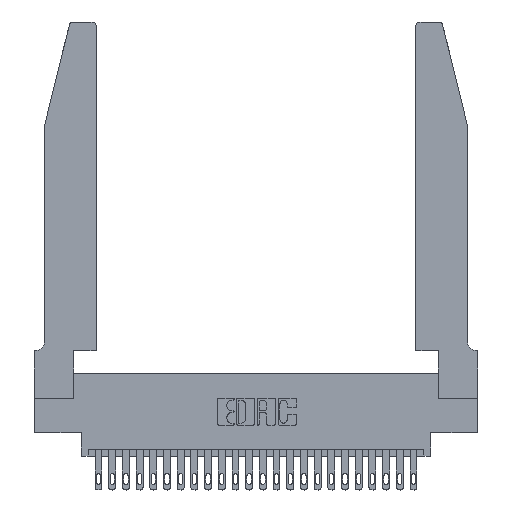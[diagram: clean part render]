
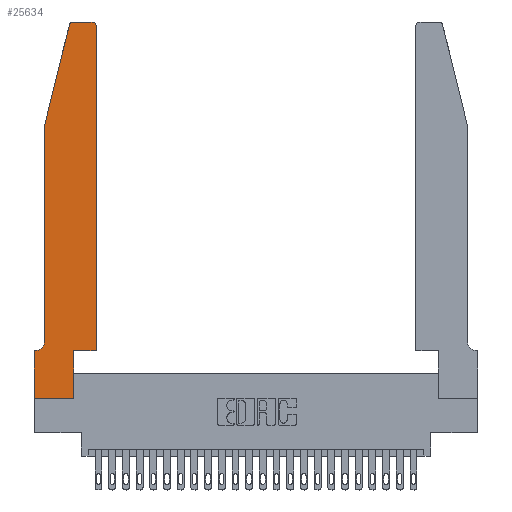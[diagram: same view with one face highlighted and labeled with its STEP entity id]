
A CAD part, top view. The second image highlights one B-rep face of the part: STEP entity #25634.
In plain terms, the highlighted planar face has unit normal (0, 0, 1).
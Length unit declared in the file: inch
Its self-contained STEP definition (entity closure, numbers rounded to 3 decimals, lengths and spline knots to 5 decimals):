
#237 = PLANE ( 'NONE',  #3318 ) ;
#264 = LINE ( 'NONE', #15603, #20413 ) ;
#269 = VERTEX_POINT ( 'NONE', #1125 ) ;
#281 = EDGE_CURVE ( 'NONE', #613, #19661, #6562, .T. ) ;
#613 = VERTEX_POINT ( 'NONE', #22108 ) ;
#935 = FACE_OUTER_BOUND ( 'NONE', #7405, .T. ) ;
#1125 = CARTESIAN_POINT ( 'NONE',  ( 0.2865, 0.35, 0.37 ) ) ;
#1539 = ORIENTED_EDGE ( 'NONE', *, *, #22946, .T. ) ;
#1851 = DIRECTION ( 'NONE',  ( -1., 0., 0. ) ) ;
#2053 = DIRECTION ( 'NONE',  ( 0., 0., 1. ) ) ;
#2150 = ORIENTED_EDGE ( 'NONE', *, *, #3081, .T. ) ;
#2611 = CARTESIAN_POINT ( 'NONE',  ( 0.0755, 2., 0.37 ) ) ;
#2825 = ORIENTED_EDGE ( 'NONE', *, *, #23355, .T. ) ;
#2946 = ORIENTED_EDGE ( 'NONE', *, *, #10987, .T. ) ;
#3009 = LINE ( 'NONE', #14976, #14350 ) ;
#3040 = CARTESIAN_POINT ( 'NONE',  ( 0.284, 2.75, 0.37 ) ) ;
#3081 = EDGE_CURVE ( 'NONE', #9734, #613, #9890, .T. ) ;
#3318 = AXIS2_PLACEMENT_3D ( 'NONE', #22066, #2053, #14320 ) ;
#3578 = AXIS2_PLACEMENT_3D ( 'NONE', #14139, #6107, #24133 ) ;
#4298 = CARTESIAN_POINT ( 'NONE',  ( 0.4505, 0.35, 0.37 ) ) ;
#4320 = VERTEX_POINT ( 'NONE', #5995 ) ;
#5757 = CARTESIAN_POINT ( 'NONE',  ( 0., 0., 0.37 ) ) ;
#5897 = VECTOR ( 'NONE', #25447, 39.37008 ) ;
#5968 = CARTESIAN_POINT ( 'NONE',  ( 0.0055, 0.35, 0.37 ) ) ;
#5995 = CARTESIAN_POINT ( 'NONE',  ( 0.4205, 2.75, 0.37 ) ) ;
#6107 = DIRECTION ( 'NONE',  ( 0., 0., 1. ) ) ;
#6520 = VERTEX_POINT ( 'NONE', #16974 ) ;
#6562 = LINE ( 'NONE', #21381, #5897 ) ;
#7014 = CARTESIAN_POINT ( 'NONE',  ( 0.4505, 0.35, 0.37 ) ) ;
#7405 = EDGE_LOOP ( 'NONE', ( #21293, #2825, #8558, #13806, #23661, #2150, #8207, #2946, #1539, #14672, #12623, #20646 ) ) ;
#7584 = VECTOR ( 'NONE', #15638, 39.37008 ) ;
#7786 = EDGE_CURVE ( 'NONE', #4320, #25905, #8513, .T. ) ;
#8207 = ORIENTED_EDGE ( 'NONE', *, *, #281, .T. ) ;
#8513 = LINE ( 'NONE', #11263, #7584 ) ;
#8558 = ORIENTED_EDGE ( 'NONE', *, *, #9553, .T. ) ;
#8597 = VERTEX_POINT ( 'NONE', #7014 ) ;
#9157 = VECTOR ( 'NONE', #10166, 39.37008 ) ;
#9553 = EDGE_CURVE ( 'NONE', #6520, #25747, #24157, .T. ) ;
#9712 = VECTOR ( 'NONE', #20358, 39.37008 ) ;
#9734 = VERTEX_POINT ( 'NONE', #5968 ) ;
#9854 = CIRCLE ( 'NONE', #3578, 0.03 ) ;
#9890 = LINE ( 'NONE', #16036, #25674 ) ;
#10166 = DIRECTION ( 'NONE',  ( 1., 0., 0. ) ) ;
#10687 = CARTESIAN_POINT ( 'NONE',  ( 0., 0., 0.37 ) ) ;
#10987 = EDGE_CURVE ( 'NONE', #19661, #14257, #15759, .T. ) ;
#11263 = CARTESIAN_POINT ( 'NONE',  ( 0.2605, 2.75, 0.37 ) ) ;
#11328 = DIRECTION ( 'NONE',  ( 1., 0., 0. ) ) ;
#11363 = AXIS2_PLACEMENT_3D ( 'NONE', #18266, #20038, #16056 ) ;
#12623 = ORIENTED_EDGE ( 'NONE', *, *, #13903, .T. ) ;
#13806 = ORIENTED_EDGE ( 'NONE', *, *, #18189, .T. ) ;
#13903 = EDGE_CURVE ( 'NONE', #8597, #25270, #25389, .T. ) ;
#13929 = LINE ( 'NONE', #21529, #23694 ) ;
#14139 = CARTESIAN_POINT ( 'NONE',  ( 0.4205, 2.72, 0.37 ) ) ;
#14220 = CARTESIAN_POINT ( 'NONE',  ( 0.2865, 0., 0.37 ) ) ;
#14257 = VERTEX_POINT ( 'NONE', #14220 ) ;
#14320 = DIRECTION ( 'NONE',  ( 1., 0., 0. ) ) ;
#14350 = VECTOR ( 'NONE', #24828, 39.37008 ) ;
#14672 = ORIENTED_EDGE ( 'NONE', *, *, #24158, .T. ) ;
#14715 = DIRECTION ( 'NONE',  ( 0., 0., 1. ) ) ;
#14976 = CARTESIAN_POINT ( 'NONE',  ( 0.0755, 2., 0.37 ) ) ;
#15603 = CARTESIAN_POINT ( 'NONE',  ( 0.2865, 0.35, 0.37 ) ) ;
#15638 = DIRECTION ( 'NONE',  ( -1., 0., 0. ) ) ;
#15759 = LINE ( 'NONE', #5757, #9157 ) ;
#16036 = CARTESIAN_POINT ( 'NONE',  ( 0.0755, 0.35, 0.37 ) ) ;
#16056 = DIRECTION ( 'NONE',  ( -1., 0., 0. ) ) ;
#16830 = CARTESIAN_POINT ( 'NONE',  ( 0.284, 2.72, 0.37 ) ) ;
#16974 = CARTESIAN_POINT ( 'NONE',  ( 0.25487, 2.72718, 0.37 ) ) ;
#17613 = DIRECTION ( 'NONE',  ( 0., 1., 0. ) ) ;
#17687 = VERTEX_POINT ( 'NONE', #22600 ) ;
#18189 = EDGE_CURVE ( 'NONE', #25747, #17687, #3009, .T. ) ;
#18266 = CARTESIAN_POINT ( 'NONE',  ( 0.0055, 0.42, 0.37 ) ) ;
#18784 = VECTOR ( 'NONE', #22741, 39.37008 ) ;
#18789 = DIRECTION ( 'NONE',  ( 1., 0., 0. ) ) ;
#18876 = CIRCLE ( 'NONE', #21344, 0.03 ) ;
#19225 = CARTESIAN_POINT ( 'NONE',  ( 0.4505, 2.72, 0.37 ) ) ;
#19320 = CIRCLE ( 'NONE', #11363, 0.07 ) ;
#19661 = VERTEX_POINT ( 'NONE', #10687 ) ;
#20038 = DIRECTION ( 'NONE',  ( 0., 0., -1. ) ) ;
#20358 = DIRECTION ( 'NONE',  ( -0.239, -0.971, 0. ) ) ;
#20413 = VECTOR ( 'NONE', #17613, 39.37008 ) ;
#20646 = ORIENTED_EDGE ( 'NONE', *, *, #20712, .T. ) ;
#20712 = EDGE_CURVE ( 'NONE', #25270, #4320, #9854, .T. ) ;
#20800 = EDGE_CURVE ( 'NONE', #17687, #9734, #19320, .T. ) ;
#21293 = ORIENTED_EDGE ( 'NONE', *, *, #7786, .T. ) ;
#21344 = AXIS2_PLACEMENT_3D ( 'NONE', #16830, #14715, #18789 ) ;
#21381 = CARTESIAN_POINT ( 'NONE',  ( 0., 0., 0.37 ) ) ;
#21529 = CARTESIAN_POINT ( 'NONE',  ( 0.4505, 0.35, 0.37 ) ) ;
#22066 = CARTESIAN_POINT ( 'NONE',  ( 0., 0.35, 0.37 ) ) ;
#22108 = CARTESIAN_POINT ( 'NONE',  ( 0., 0.35, 0.37 ) ) ;
#22600 = CARTESIAN_POINT ( 'NONE',  ( 0.0755, 0.42, 0.37 ) ) ;
#22701 = CARTESIAN_POINT ( 'NONE',  ( 0.0755, 2., 0.37 ) ) ;
#22741 = DIRECTION ( 'NONE',  ( 0., 1., 0. ) ) ;
#22946 = EDGE_CURVE ( 'NONE', #14257, #269, #264, .T. ) ;
#23355 = EDGE_CURVE ( 'NONE', #25905, #6520, #18876, .T. ) ;
#23661 = ORIENTED_EDGE ( 'NONE', *, *, #20800, .T. ) ;
#23694 = VECTOR ( 'NONE', #11328, 39.37008 ) ;
#24133 = DIRECTION ( 'NONE',  ( 1., 0., 0. ) ) ;
#24157 = LINE ( 'NONE', #2611, #9712 ) ;
#24158 = EDGE_CURVE ( 'NONE', #269, #8597, #13929, .T. ) ;
#24828 = DIRECTION ( 'NONE',  ( 0., -1., 0. ) ) ;
#25270 = VERTEX_POINT ( 'NONE', #19225 ) ;
#25389 = LINE ( 'NONE', #4298, #18784 ) ;
#25447 = DIRECTION ( 'NONE',  ( 0., -1., 0. ) ) ;
#25634 = ADVANCED_FACE ( 'NONE', ( #935 ), #237, .T. ) ;
#25674 = VECTOR ( 'NONE', #1851, 39.37008 ) ;
#25747 = VERTEX_POINT ( 'NONE', #22701 ) ;
#25905 = VERTEX_POINT ( 'NONE', #3040 ) ;
